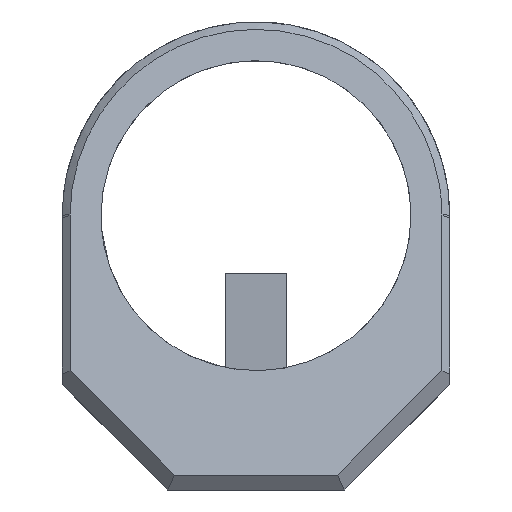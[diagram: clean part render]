
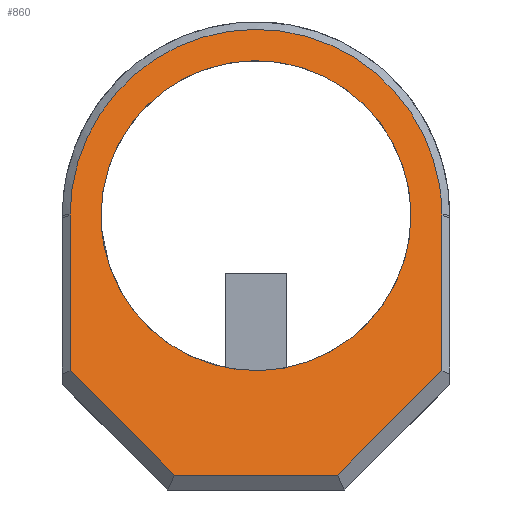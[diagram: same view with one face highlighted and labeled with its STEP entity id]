
A CAD part, left-side view. The second image highlights one B-rep face of the part: STEP entity #860.
In plain terms, the highlighted planar face has unit normal (-0.966, 0, 0.259).
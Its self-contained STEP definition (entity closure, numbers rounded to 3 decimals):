
#24=B_SPLINE_CURVE_WITH_KNOTS('',3,(#1295,#1296,#1297,#1298,#1299,#1300,
#1301,#1302,#1303,#1304),.UNSPECIFIED.,.F.,.F.,(4,1,1,1,1,1,1,4),(-1.56,
-1.115,-0.669,-0.223,0.223,
0.669,1.115,1.56),.UNSPECIFIED.);
#27=B_SPLINE_CURVE_WITH_KNOTS('',3,(#1337,#1338,#1339,#1340),
 .UNSPECIFIED.,.F.,.F.,(4,4),(-1.571,-1.56),
 .UNSPECIFIED.);
#29=B_SPLINE_CURVE_WITH_KNOTS('',3,(#1380,#1381,#1382,#1383),
 .UNSPECIFIED.,.F.,.F.,(4,4),(1.56,1.571),
 .UNSPECIFIED.);
#35=FACE_BOUND('',#122,.T.);
#74=FACE_OUTER_BOUND('',#121,.T.);
#121=EDGE_LOOP('',(#712,#713,#714,#715,#716,#717,#718,#719));
#122=EDGE_LOOP('',(#720));
#171=LINE('',#1235,#273);
#178=LINE('',#1249,#280);
#182=LINE('',#1344,#284);
#190=LINE('',#1359,#292);
#212=LINE('',#1512,#314);
#273=VECTOR('',#1004,10.);
#280=VECTOR('',#1013,10.);
#284=VECTOR('',#1019,10.);
#292=VECTOR('',#1029,10.);
#314=VECTOR('',#1073,10.);
#344=ELLIPSE('',#895,5.176,5.);
#356=VERTEX_POINT('',#1159);
#380=VERTEX_POINT('',#1233);
#381=VERTEX_POINT('',#1234);
#387=VERTEX_POINT('',#1247);
#389=VERTEX_POINT('',#1292);
#390=VERTEX_POINT('',#1294);
#392=VERTEX_POINT('',#1342);
#393=VERTEX_POINT('',#1343);
#399=VERTEX_POINT('',#1357);
#439=EDGE_CURVE('',#356,#356,#344,.T.);
#469=EDGE_CURVE('',#380,#381,#171,.T.);
#476=EDGE_CURVE('',#387,#380,#178,.T.);
#479=EDGE_CURVE('',#389,#390,#24,.T.);
#483=EDGE_CURVE('',#381,#389,#27,.T.);
#484=EDGE_CURVE('',#392,#393,#182,.T.);
#492=EDGE_CURVE('',#399,#392,#190,.T.);
#494=EDGE_CURVE('',#390,#399,#29,.T.);
#520=EDGE_CURVE('',#393,#387,#212,.T.);
#712=ORIENTED_EDGE('',*,*,#476,.F.);
#713=ORIENTED_EDGE('',*,*,#520,.F.);
#714=ORIENTED_EDGE('',*,*,#484,.F.);
#715=ORIENTED_EDGE('',*,*,#492,.F.);
#716=ORIENTED_EDGE('',*,*,#494,.F.);
#717=ORIENTED_EDGE('',*,*,#479,.F.);
#718=ORIENTED_EDGE('',*,*,#483,.F.);
#719=ORIENTED_EDGE('',*,*,#469,.F.);
#720=ORIENTED_EDGE('',*,*,#439,.T.);
#816=PLANE('',#920);
#860=ADVANCED_FACE('',(#74,#35),#816,.T.);
#895=AXIS2_PLACEMENT_3D('',#1160,#960,#961);
#920=AXIS2_PLACEMENT_3D('',#1513,#1074,#1075);
#960=DIRECTION('center_axis',(0.966,0.,-0.259));
#961=DIRECTION('ref_axis',(-0.259,0.,-0.966));
#1004=DIRECTION('',(0.259,0.,0.966));
#1013=DIRECTION('',(0.186,0.695,0.695));
#1019=DIRECTION('',(-0.186,0.695,-0.695));
#1029=DIRECTION('',(-0.259,0.,-0.966));
#1073=DIRECTION('',(0.,1.,0.));
#1074=DIRECTION('center_axis',(-0.966,0.,0.259));
#1075=DIRECTION('ref_axis',(0.,-1.,0.));
#1159=CARTESIAN_POINT('',(2.371,-36.25,5.45));
#1160=CARTESIAN_POINT('Origin',(2.371,-41.25,5.45));
#1233=CARTESIAN_POINT('',(1.03,-35.25,0.445));
#1234=CARTESIAN_POINT('',(2.371,-35.25,5.45));
#1235=CARTESIAN_POINT('',(0.865,-35.25,-0.172));
#1247=CARTESIAN_POINT('',(0.129,-38.612,-2.917));
#1249=CARTESIAN_POINT('',(1.279,-34.321,1.374));
#1292=CARTESIAN_POINT('',(2.388,-35.25,5.512));
#1294=CARTESIAN_POINT('',(2.388,-47.25,5.512));
#1295=CARTESIAN_POINT('Ctrl Pts',(2.388,-35.25,5.512));
#1296=CARTESIAN_POINT('Ctrl Pts',(2.628,-35.26,6.406));
#1297=CARTESIAN_POINT('Ctrl Pts',(3.105,-35.684,8.19));
#1298=CARTESIAN_POINT('Ctrl Pts',(3.678,-37.408,10.326));
#1299=CARTESIAN_POINT('Ctrl Pts',(3.995,-39.881,11.508));
#1300=CARTESIAN_POINT('Ctrl Pts',(3.994,-42.619,11.507));
#1301=CARTESIAN_POINT('Ctrl Pts',(3.678,-45.092,10.327));
#1302=CARTESIAN_POINT('Ctrl Pts',(3.105,-46.816,8.19));
#1303=CARTESIAN_POINT('Ctrl Pts',(2.628,-47.24,6.406));
#1304=CARTESIAN_POINT('Ctrl Pts',(2.388,-47.25,5.512));
#1337=CARTESIAN_POINT('Ctrl Pts',(2.371,-35.25,5.45));
#1338=CARTESIAN_POINT('Ctrl Pts',(2.377,-35.25,5.471));
#1339=CARTESIAN_POINT('Ctrl Pts',(2.382,-35.25,5.492));
#1340=CARTESIAN_POINT('Ctrl Pts',(2.388,-35.25,5.512));
#1342=CARTESIAN_POINT('',(1.03,-47.25,0.445));
#1343=CARTESIAN_POINT('',(0.129,-43.888,-2.917));
#1344=CARTESIAN_POINT('',(0.471,-45.162,-1.643));
#1357=CARTESIAN_POINT('',(2.371,-47.25,5.45));
#1359=CARTESIAN_POINT('',(2.315,-47.25,5.24));
#1380=CARTESIAN_POINT('Ctrl Pts',(2.388,-47.25,5.512));
#1381=CARTESIAN_POINT('Ctrl Pts',(2.382,-47.25,5.492));
#1382=CARTESIAN_POINT('Ctrl Pts',(2.377,-47.25,5.471));
#1383=CARTESIAN_POINT('Ctrl Pts',(2.371,-47.25,5.45));
#1512=CARTESIAN_POINT('',(0.129,-38.125,-2.917));
#1513=CARTESIAN_POINT('Origin',(0.88,-35.,-0.116));
